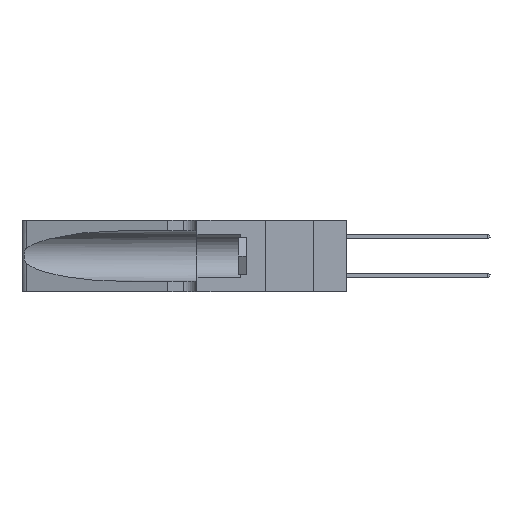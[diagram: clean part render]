
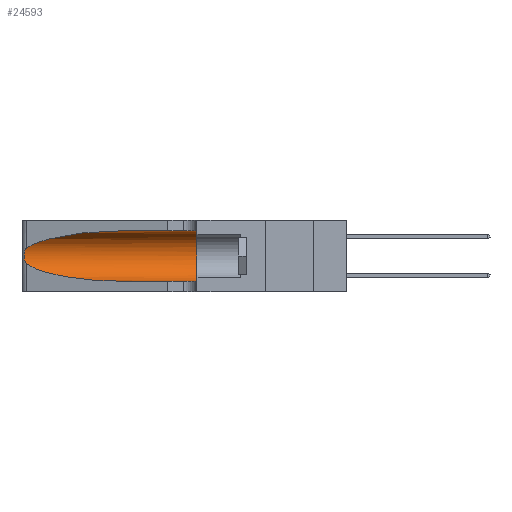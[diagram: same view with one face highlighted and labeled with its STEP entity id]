
A CAD part, left-side view. The second image highlights one B-rep face of the part: STEP entity #24593.
In plain terms, the highlighted cylindrical face has radius 3.308 mm (diameter 6.617 mm), a partial arc.
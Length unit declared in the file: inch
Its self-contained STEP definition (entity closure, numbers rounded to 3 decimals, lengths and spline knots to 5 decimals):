
#447 = VECTOR ( 'NONE', #25782, 39.37008 ) ;
#1745 = VERTEX_POINT ( 'NONE', #19007 ) ;
#2170 = CARTESIAN_POINT ( 'NONE',  ( 0.26075, 1.23896, 0.19203 ) ) ;
#2638 = CARTESIAN_POINT ( 'NONE',  ( 0.25487, 1.22718, 0.22369 ) ) ;
#3018 = ORIENTED_EDGE ( 'NONE', *, *, #25621, .T. ) ;
#4514 = EDGE_CURVE ( 'NONE', #13732, #21467, #10114, .T. ) ;
#4560 = CARTESIAN_POINT ( 'NONE',  ( 0.2373, 1.15595, 0.08982 ) ) ;
#4659 = ORIENTED_EDGE ( 'NONE', *, *, #26661, .T. ) ;
#4692 = CARTESIAN_POINT ( 'NONE',  ( 0.26017, 1.23833, 0.17102 ) ) ;
#5431 = CARTESIAN_POINT ( 'NONE',  ( 0.1305, 0.35, 0.185 ) ) ;
#5921 = ORIENTED_EDGE ( 'NONE', *, *, #16790, .T. ) ;
#6030 = CARTESIAN_POINT ( 'NONE',  ( 0.1305, 1.61858, 0.05475 ) ) ;
#6414 =( BOUNDED_CURVE ( )  B_SPLINE_CURVE ( 3, ( #19424, #4560, #21892, #7032 ),
 .UNSPECIFIED., .F., .F. ) 
 B_SPLINE_CURVE_WITH_KNOTS ( ( 4, 4 ),
 ( 3.44316, 4.71239 ),
 .UNSPECIFIED. ) 
 CURVE ( )  GEOMETRIC_REPRESENTATION_ITEM ( )  RATIONAL_B_SPLINE_CURVE ( ( 1., 0.87, 0.87, 1. ) ) 
 REPRESENTATION_ITEM ( '' )  );
#7032 = CARTESIAN_POINT ( 'NONE',  ( 0.1305, 0.72297, 0.05475 ) ) ;
#7058 = CARTESIAN_POINT ( 'NONE',  ( 0.25555, 1.22994, 0.2215 ) ) ;
#7165 = CARTESIAN_POINT ( 'NONE',  ( 0.25789, 1.23486, 0.15765 ) ) ;
#7940 = DIRECTION ( 'NONE',  ( 0., 0., 1. ) ) ;
#8223 = CARTESIAN_POINT ( 'NONE',  ( 0.1305, 1.61858, 0.31525 ) ) ;
#9618 = CARTESIAN_POINT ( 'NONE',  ( 0.1305, 1.61858, 0.185 ) ) ;
#9701 = CARTESIAN_POINT ( 'NONE',  ( 0.25555, 1.22993, 0.14849 ) ) ;
#10114 = LINE ( 'NONE', #8223, #22465 ) ;
#10614 = EDGE_CURVE ( 'NONE', #21467, #17147, #22005, .T. ) ;
#12031 = CARTESIAN_POINT ( 'NONE',  ( 0.25487, 1.22718, 0.14631 ) ) ;
#12105 = DIRECTION ( 'NONE',  ( 0., 0., -1. ) ) ;
#12255 =( BOUNDED_CURVE ( )  B_SPLINE_CURVE ( 3, ( #15033, #22360, #17504, #2638 ),
 .UNSPECIFIED., .F., .F. ) 
 B_SPLINE_CURVE_WITH_KNOTS ( ( 4, 4 ),
 ( 1.5708, 2.84003 ),
 .UNSPECIFIED. ) 
 CURVE ( )  GEOMETRIC_REPRESENTATION_ITEM ( )  RATIONAL_B_SPLINE_CURVE ( ( 1., 0.87, 0.87, 1. ) ) 
 REPRESENTATION_ITEM ( '' )  );
#12806 = CARTESIAN_POINT ( 'NONE',  ( 0.25487, 1.22718, 0.22369 ) ) ;
#12929 = AXIS2_PLACEMENT_3D ( 'NONE', #9618, #26844, #12105 ) ;
#13235 = DIRECTION ( 'NONE',  ( 0., -1., 0. ) ) ;
#13732 = VERTEX_POINT ( 'NONE', #26434 ) ;
#14576 = CARTESIAN_POINT ( 'NONE',  ( 0.25787, 1.23484, 0.2124 ) ) ;
#15033 = CARTESIAN_POINT ( 'NONE',  ( 0.1305, 0.72297, 0.31525 ) ) ;
#15403 = FACE_OUTER_BOUND ( 'NONE', #29868, .T. ) ;
#16208 = VERTEX_POINT ( 'NONE', #12806 ) ;
#16292 = CARTESIAN_POINT ( 'NONE',  ( 0.1305, 0.35, 0.05475 ) ) ;
#16617 = VERTEX_POINT ( 'NONE', #12031 ) ;
#16790 = EDGE_CURVE ( 'NONE', #13732, #16208, #12255, .T. ) ;
#16832 = ORIENTED_EDGE ( 'NONE', *, *, #10614, .F. ) ;
#17047 = CARTESIAN_POINT ( 'NONE',  ( 0.26018, 1.23835, 0.19895 ) ) ;
#17147 = VERTEX_POINT ( 'NONE', #16292 ) ;
#17504 = CARTESIAN_POINT ( 'NONE',  ( 0.2373, 1.15595, 0.28018 ) ) ;
#18893 = AXIS2_PLACEMENT_3D ( 'NONE', #5431, #22740, #7940 ) ;
#19007 = CARTESIAN_POINT ( 'NONE',  ( 0.1305, 0.72297, 0.05475 ) ) ;
#19192 = EDGE_CURVE ( 'NONE', #16617, #1745, #6414, .T. ) ;
#19424 = CARTESIAN_POINT ( 'NONE',  ( 0.25487, 1.22718, 0.14631 ) ) ;
#19546 = CARTESIAN_POINT ( 'NONE',  ( 0.26075, 1.23896, 0.178 ) ) ;
#20442 = CYLINDRICAL_SURFACE ( 'NONE', #12929, 0.13025 ) ;
#21247 = ORIENTED_EDGE ( 'NONE', *, *, #19192, .T. ) ;
#21467 = VERTEX_POINT ( 'NONE', #22984 ) ;
#21892 = CARTESIAN_POINT ( 'NONE',  ( 0.18966, 0.96281, 0.05475 ) ) ;
#22005 = CIRCLE ( 'NONE', #18893, 0.13025 ) ;
#22021 = CARTESIAN_POINT ( 'NONE',  ( 0.25856, 1.23593, 0.16098 ) ) ;
#22360 = CARTESIAN_POINT ( 'NONE',  ( 0.18966, 0.96281, 0.31525 ) ) ;
#22465 = VECTOR ( 'NONE', #13235, 39.37008 ) ;
#22740 = DIRECTION ( 'NONE',  ( 0., 1., 0. ) ) ;
#22984 = CARTESIAN_POINT ( 'NONE',  ( 0.1305, 0.35, 0.31525 ) ) ;
#24233 = CARTESIAN_POINT ( 'NONE',  ( 0.25487, 1.22718, 0.22369 ) ) ;
#24438 = CARTESIAN_POINT ( 'NONE',  ( 0.25639, 1.23186, 0.15144 ) ) ;
#24593 = ADVANCED_FACE ( 'NONE', ( #15403 ), #20442, .F. ) ;
#25621 = EDGE_CURVE ( 'NONE', #1745, #17147, #26855, .T. ) ;
#25782 = DIRECTION ( 'NONE',  ( 0., -1., 0. ) ) ;
#26434 = CARTESIAN_POINT ( 'NONE',  ( 0.1305, 0.72297, 0.31525 ) ) ;
#26661 = EDGE_CURVE ( 'NONE', #16208, #16617, #27045, .T. ) ;
#26844 = DIRECTION ( 'NONE',  ( 0., -1., 0. ) ) ;
#26855 = LINE ( 'NONE', #6030, #447 ) ;
#26934 = CARTESIAN_POINT ( 'NONE',  ( 0.25487, 1.22718, 0.14631 ) ) ;
#27045 = B_SPLINE_CURVE_WITH_KNOTS ( 'NONE', 3,
 ( #24233, #7058, #29298, #14576, #31708, #17047, #2170, #19546, #4692, #22021, #7165, #24438, #9701, #26934 ),
 .UNSPECIFIED., .F., .F.,
 ( 4, 2, 2, 2, 2, 2, 4 ),
 ( 0., 0.00027, 0.00053, 0.00107, 0.0016, 0.00187, 0.00214 ),
 .UNSPECIFIED. ) ;
#29298 = CARTESIAN_POINT ( 'NONE',  ( 0.25639, 1.23184, 0.21858 ) ) ;
#29868 = EDGE_LOOP ( 'NONE', ( #5921, #4659, #21247, #3018, #16832, #30137 ) ) ;
#30137 = ORIENTED_EDGE ( 'NONE', *, *, #4514, .F. ) ;
#31708 = CARTESIAN_POINT ( 'NONE',  ( 0.25854, 1.2359, 0.20912 ) ) ;
